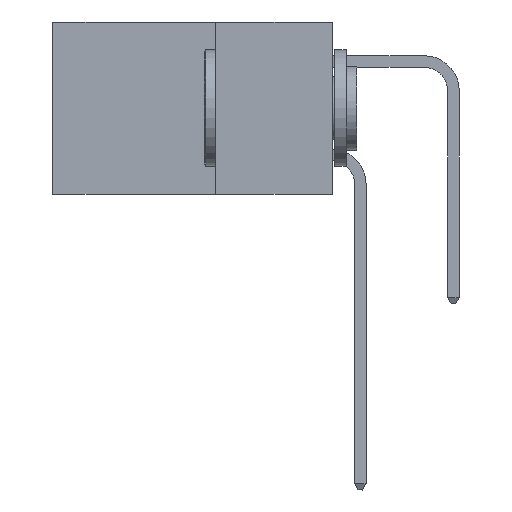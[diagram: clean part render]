
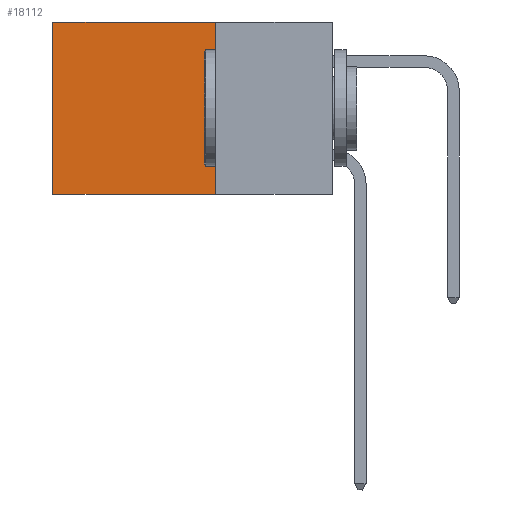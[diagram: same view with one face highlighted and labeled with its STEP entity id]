
A CAD part, left-side view. The second image highlights one B-rep face of the part: STEP entity #18112.
In plain terms, the highlighted planar face has unit normal (-1, 0, 0).
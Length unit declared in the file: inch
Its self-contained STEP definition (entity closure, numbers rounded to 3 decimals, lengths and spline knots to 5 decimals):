
#985 = VECTOR ( 'NONE', #19870, 39.37008 ) ;
#1315 = CARTESIAN_POINT ( 'NONE',  ( 0.298, 0.6, -0.37 ) ) ;
#1959 = DIRECTION ( 'NONE',  ( 0., 1., 0. ) ) ;
#2883 = EDGE_CURVE ( 'NONE', #10940, #10851, #12941, .T. ) ;
#3603 = DIRECTION ( 'NONE',  ( 0., 1., 0. ) ) ;
#4011 = VECTOR ( 'NONE', #3603, 39.37008 ) ;
#4107 = CARTESIAN_POINT ( 'NONE',  ( 0.298, 0.6, 0. ) ) ;
#4427 = ORIENTED_EDGE ( 'NONE', *, *, #27647, .T. ) ;
#4925 = VERTEX_POINT ( 'NONE', #15329 ) ;
#6788 = PLANE ( 'NONE',  #11524 ) ;
#7946 = VERTEX_POINT ( 'NONE', #19512 ) ;
#9253 = DIRECTION ( 'NONE',  ( 1., 0., 0. ) ) ;
#10302 = LINE ( 'NONE', #13816, #27515 ) ;
#10436 = LINE ( 'NONE', #29442, #4011 ) ;
#10851 = VERTEX_POINT ( 'NONE', #1315 ) ;
#10940 = VERTEX_POINT ( 'NONE', #4107 ) ;
#11524 = AXIS2_PLACEMENT_3D ( 'NONE', #23288, #9253, #25690 ) ;
#11559 = ORIENTED_EDGE ( 'NONE', *, *, #19094, .F. ) ;
#12941 = LINE ( 'NONE', #19932, #985 ) ;
#13816 = CARTESIAN_POINT ( 'NONE',  ( 0.298, 0.25, 0. ) ) ;
#15329 = CARTESIAN_POINT ( 'NONE',  ( 0.298, 0.25, 0. ) ) ;
#15714 = VECTOR ( 'NONE', #19537, 39.37008 ) ;
#16048 = EDGE_CURVE ( 'NONE', #4925, #7946, #16469, .T. ) ;
#16469 = LINE ( 'NONE', #17168, #15714 ) ;
#17168 = CARTESIAN_POINT ( 'NONE',  ( 0.298, 0.25, 0. ) ) ;
#18112 = ADVANCED_FACE ( 'NONE', ( #26636 ), #6788, .F. ) ;
#18902 = ORIENTED_EDGE ( 'NONE', *, *, #16048, .F. ) ;
#19094 = EDGE_CURVE ( 'NONE', #7946, #10851, #10436, .T. ) ;
#19512 = CARTESIAN_POINT ( 'NONE',  ( 0.298, 0.25, -0.37 ) ) ;
#19537 = DIRECTION ( 'NONE',  ( 0., 0., -1. ) ) ;
#19870 = DIRECTION ( 'NONE',  ( 0., 0., -1. ) ) ;
#19932 = CARTESIAN_POINT ( 'NONE',  ( 0.298, 0.6, 0. ) ) ;
#20523 = ORIENTED_EDGE ( 'NONE', *, *, #2883, .T. ) ;
#20717 = EDGE_LOOP ( 'NONE', ( #20523, #11559, #18902, #4427 ) ) ;
#23288 = CARTESIAN_POINT ( 'NONE',  ( 0.298, 0.25, 0. ) ) ;
#25690 = DIRECTION ( 'NONE',  ( 0., 0., -1. ) ) ;
#26636 = FACE_OUTER_BOUND ( 'NONE', #20717, .T. ) ;
#27515 = VECTOR ( 'NONE', #1959, 39.37008 ) ;
#27647 = EDGE_CURVE ( 'NONE', #4925, #10940, #10302, .T. ) ;
#29442 = CARTESIAN_POINT ( 'NONE',  ( 0.298, 0.25, -0.37 ) ) ;
